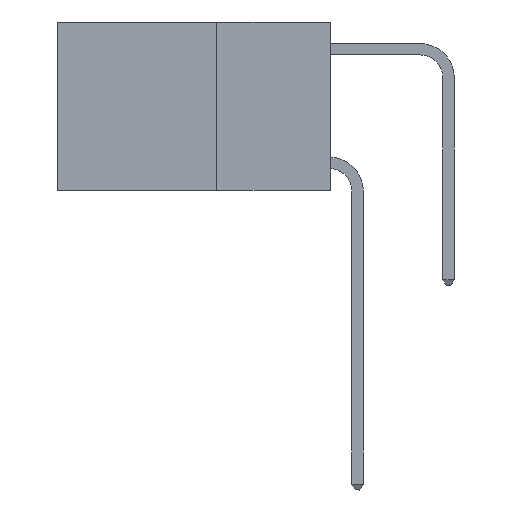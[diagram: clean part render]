
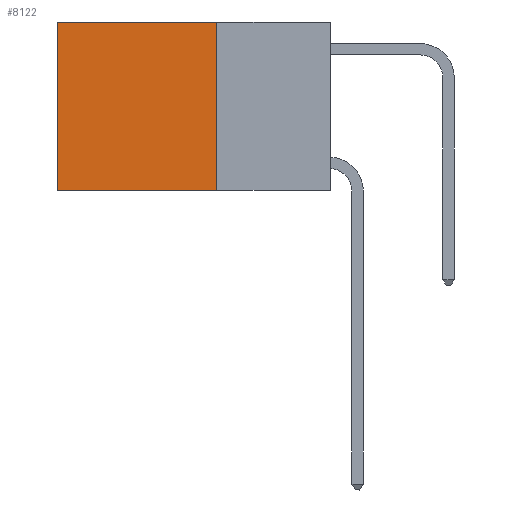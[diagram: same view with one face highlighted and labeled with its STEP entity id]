
A CAD part, left-side view. The second image highlights one B-rep face of the part: STEP entity #8122.
In plain terms, the highlighted planar face has unit normal (-1, 0, 0).
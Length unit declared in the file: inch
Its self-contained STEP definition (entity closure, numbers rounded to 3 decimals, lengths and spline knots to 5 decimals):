
#585 = ORIENTED_EDGE ( 'NONE', *, *, #2014, .F. ) ;
#938 = CARTESIAN_POINT ( 'NONE',  ( 0.2625, 0.6, -0.37 ) ) ;
#1438 = ORIENTED_EDGE ( 'NONE', *, *, #5043, .T. ) ;
#1537 = ORIENTED_EDGE ( 'NONE', *, *, #4276, .T. ) ;
#1577 = ORIENTED_EDGE ( 'NONE', *, *, #6014, .F. ) ;
#1598 = EDGE_LOOP ( 'NONE', ( #1537, #585, #1577, #1438 ) ) ;
#1855 = DIRECTION ( 'NONE',  ( 0., 0., -1. ) ) ;
#2014 = EDGE_CURVE ( 'NONE', #11321, #10450, #2050, .T. ) ;
#2050 = LINE ( 'NONE', #9294, #8643 ) ;
#2157 = VERTEX_POINT ( 'NONE', #4800 ) ;
#2183 = VECTOR ( 'NONE', #1855, 39.37008 ) ;
#2655 = CARTESIAN_POINT ( 'NONE',  ( 0.2625, 0.25, 0. ) ) ;
#3630 = AXIS2_PLACEMENT_3D ( 'NONE', #11094, #10221, #5763 ) ;
#4276 = EDGE_CURVE ( 'NONE', #2157, #10450, #11525, .T. ) ;
#4477 = DIRECTION ( 'NONE',  ( 0., 0., -1. ) ) ;
#4800 = CARTESIAN_POINT ( 'NONE',  ( 0.2625, 0.6, 0. ) ) ;
#5043 = EDGE_CURVE ( 'NONE', #10714, #2157, #9512, .T. ) ;
#5415 = CARTESIAN_POINT ( 'NONE',  ( 0.2625, 0.6, 0. ) ) ;
#5763 = DIRECTION ( 'NONE',  ( 0., 0., -1. ) ) ;
#6014 = EDGE_CURVE ( 'NONE', #10714, #11321, #6630, .T. ) ;
#6176 = VECTOR ( 'NONE', #11432, 39.37008 ) ;
#6630 = LINE ( 'NONE', #11397, #7726 ) ;
#7726 = VECTOR ( 'NONE', #4477, 39.37008 ) ;
#8122 = ADVANCED_FACE ( 'NONE', ( #11420 ), #8442, .F. ) ;
#8419 = DIRECTION ( 'NONE',  ( 0., 1., 0. ) ) ;
#8442 = PLANE ( 'NONE',  #3630 ) ;
#8643 = VECTOR ( 'NONE', #8419, 39.37008 ) ;
#9294 = CARTESIAN_POINT ( 'NONE',  ( 0.2625, 0.25, -0.37 ) ) ;
#9464 = CARTESIAN_POINT ( 'NONE',  ( 0.2625, 0.25, -0.37 ) ) ;
#9496 = CARTESIAN_POINT ( 'NONE',  ( 0.2625, 0.25, 0. ) ) ;
#9512 = LINE ( 'NONE', #2655, #6176 ) ;
#10221 = DIRECTION ( 'NONE',  ( 1., 0., 0. ) ) ;
#10450 = VERTEX_POINT ( 'NONE', #938 ) ;
#10714 = VERTEX_POINT ( 'NONE', #9496 ) ;
#11094 = CARTESIAN_POINT ( 'NONE',  ( 0.2625, 0.25, 0. ) ) ;
#11321 = VERTEX_POINT ( 'NONE', #9464 ) ;
#11397 = CARTESIAN_POINT ( 'NONE',  ( 0.2625, 0.25, 0. ) ) ;
#11420 = FACE_OUTER_BOUND ( 'NONE', #1598, .T. ) ;
#11432 = DIRECTION ( 'NONE',  ( 0., 1., 0. ) ) ;
#11525 = LINE ( 'NONE', #5415, #2183 ) ;
